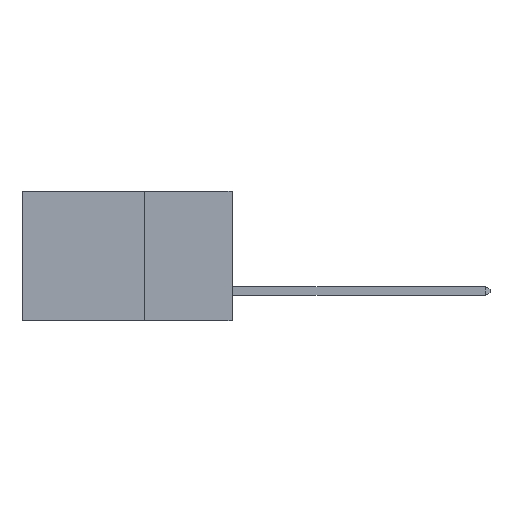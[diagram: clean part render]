
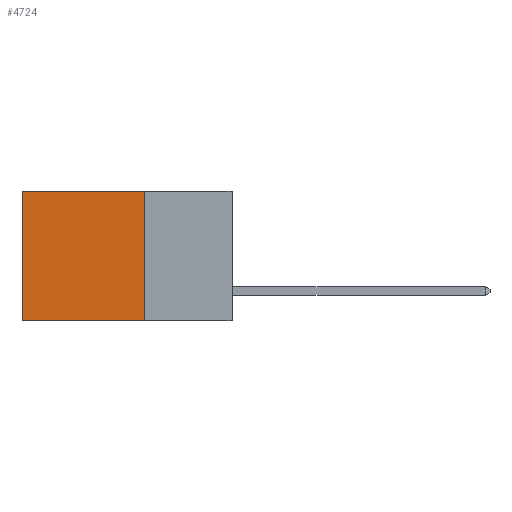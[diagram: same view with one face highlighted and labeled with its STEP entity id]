
A CAD part, left-side view. The second image highlights one B-rep face of the part: STEP entity #4724.
In plain terms, the highlighted planar face has unit normal (-1, 0, 0).
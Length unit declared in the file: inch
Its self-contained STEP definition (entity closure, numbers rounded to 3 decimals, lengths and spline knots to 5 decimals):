
#1199 = ORIENTED_EDGE ( 'NONE', *, *, #11322, .F. ) ;
#1447 = VECTOR ( 'NONE', #5913, 39.37008 ) ;
#2370 = VECTOR ( 'NONE', #10578, 39.37008 ) ;
#3792 = EDGE_CURVE ( 'NONE', #4719, #14401, #12176, .T. ) ;
#4555 = ORIENTED_EDGE ( 'NONE', *, *, #7326, .T. ) ;
#4719 = VERTEX_POINT ( 'NONE', #13306 ) ;
#4724 = ADVANCED_FACE ( 'NONE', ( #10953 ), #16401, .F. ) ;
#5727 = EDGE_LOOP ( 'NONE', ( #6281, #1199, #15107, #4555 ) ) ;
#5913 = DIRECTION ( 'NONE',  ( 0., 1., 0. ) ) ;
#6281 = ORIENTED_EDGE ( 'NONE', *, *, #19546, .T. ) ;
#7326 = EDGE_CURVE ( 'NONE', #4719, #10192, #9608, .T. ) ;
#7886 = DIRECTION ( 'NONE',  ( 0., 1., 0. ) ) ;
#8013 = VECTOR ( 'NONE', #17351, 39.37008 ) ;
#8995 = CARTESIAN_POINT ( 'NONE',  ( 0.2875, 0.6, 0. ) ) ;
#9608 = LINE ( 'NONE', #15287, #1447 ) ;
#9658 = LINE ( 'NONE', #20159, #17359 ) ;
#10192 = VERTEX_POINT ( 'NONE', #16692 ) ;
#10292 = DIRECTION ( 'NONE',  ( 0., 0., -1. ) ) ;
#10578 = DIRECTION ( 'NONE',  ( 0., 0., -1. ) ) ;
#10953 = FACE_OUTER_BOUND ( 'NONE', #5727, .T. ) ;
#11322 = EDGE_CURVE ( 'NONE', #14401, #14097, #9658, .T. ) ;
#11458 = LINE ( 'NONE', #8995, #2370 ) ;
#11776 = CARTESIAN_POINT ( 'NONE',  ( 0.2875, 0.25, 0. ) ) ;
#12176 = LINE ( 'NONE', #15821, #8013 ) ;
#13306 = CARTESIAN_POINT ( 'NONE',  ( 0.2875, 0.25, 0. ) ) ;
#14097 = VERTEX_POINT ( 'NONE', #19196 ) ;
#14401 = VERTEX_POINT ( 'NONE', #18387 ) ;
#15107 = ORIENTED_EDGE ( 'NONE', *, *, #3792, .F. ) ;
#15287 = CARTESIAN_POINT ( 'NONE',  ( 0.2875, 0.25, 0. ) ) ;
#15821 = CARTESIAN_POINT ( 'NONE',  ( 0.2875, 0.25, 0. ) ) ;
#16401 = PLANE ( 'NONE',  #16729 ) ;
#16692 = CARTESIAN_POINT ( 'NONE',  ( 0.2875, 0.6, 0. ) ) ;
#16729 = AXIS2_PLACEMENT_3D ( 'NONE', #11776, #19473, #10292 ) ;
#17351 = DIRECTION ( 'NONE',  ( 0., 0., -1. ) ) ;
#17359 = VECTOR ( 'NONE', #7886, 39.37008 ) ;
#18387 = CARTESIAN_POINT ( 'NONE',  ( 0.2875, 0.25, -0.37 ) ) ;
#19196 = CARTESIAN_POINT ( 'NONE',  ( 0.2875, 0.6, -0.37 ) ) ;
#19473 = DIRECTION ( 'NONE',  ( 1., 0., 0. ) ) ;
#19546 = EDGE_CURVE ( 'NONE', #10192, #14097, #11458, .T. ) ;
#20159 = CARTESIAN_POINT ( 'NONE',  ( 0.2875, 0.25, -0.37 ) ) ;
